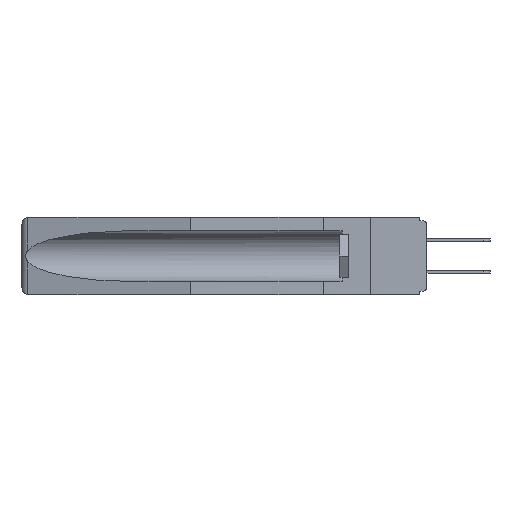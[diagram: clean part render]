
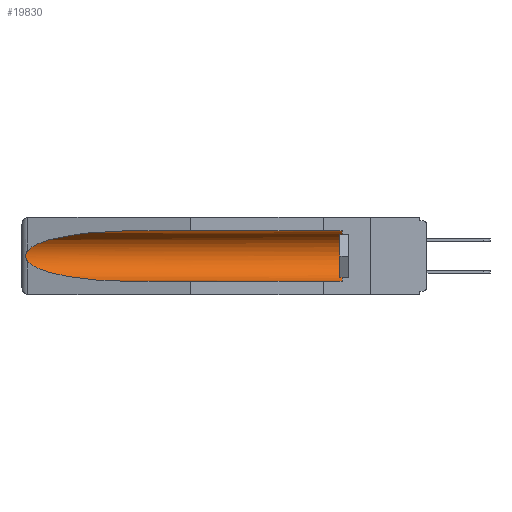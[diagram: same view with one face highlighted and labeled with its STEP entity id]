
A CAD part, left-side view. The second image highlights one B-rep face of the part: STEP entity #19830.
In plain terms, the highlighted cylindrical face has radius 2.857 mm (diameter 5.715 mm), a partial arc.
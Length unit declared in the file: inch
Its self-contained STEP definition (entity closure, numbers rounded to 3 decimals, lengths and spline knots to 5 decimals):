
#35 = CARTESIAN_POINT ( 'NONE',  ( 0.26655, 1.53094, -0.18657 ) ) ;
#414 = CYLINDRICAL_SURFACE ( 'NONE', #18750, 0.1125 ) ;
#430 = B_SPLINE_CURVE_WITH_KNOTS ( 'NONE', 3,
 ( #4669, #11144, #17852, #14540, #1374, #9643, #8009, #35, #12796, #11447 ),
 .UNSPECIFIED., .F., .F.,
 ( 4, 2, 2, 2, 4 ),
 ( 0., 0.00029, 0.00058, 0.00087, 0.00117 ),
 .UNSPECIFIED. ) ;
#1374 = CARTESIAN_POINT ( 'NONE',  ( 0.2675, 1.53308, -0.16763 ) ) ;
#1509 =( BOUNDED_CURVE ( )  B_SPLINE_CURVE ( 3, ( #13506, #6968, #18160, #20005 ),
 .UNSPECIFIED., .F., .F. ) 
 B_SPLINE_CURVE_WITH_KNOTS ( ( 4, 4 ),
 ( 4.71239, 6.08839 ),
 .UNSPECIFIED. ) 
 CURVE ( )  GEOMETRIC_REPRESENTATION_ITEM ( )  RATIONAL_B_SPLINE_CURVE ( ( 1., 0.848, 0.848, 1. ) ) 
 REPRESENTATION_ITEM ( '' )  );
#1814 = DIRECTION ( 'NONE',  ( 0., 1., 0. ) ) ;
#2579 = VERTEX_POINT ( 'NONE', #17797 ) ;
#2738 = ORIENTED_EDGE ( 'NONE', *, *, #10121, .T. ) ;
#2760 = EDGE_CURVE ( 'NONE', #20388, #2579, #17540, .T. ) ;
#4669 = CARTESIAN_POINT ( 'NONE',  ( 0.26537, 1.52718, -0.14972 ) ) ;
#5273 = ORIENTED_EDGE ( 'NONE', *, *, #15916, .F. ) ;
#5324 = DIRECTION ( 'NONE',  ( 0., 1., 0. ) ) ;
#5641 = CARTESIAN_POINT ( 'NONE',  ( 0.21114, 1.30732, -0.284 ) ) ;
#6081 = EDGE_CURVE ( 'NONE', #13293, #14736, #18174, .T. ) ;
#6417 = CARTESIAN_POINT ( 'NONE',  ( 0.26537, 1.52718, -0.14972 ) ) ;
#6472 = DIRECTION ( 'NONE',  ( 0., 0., 1. ) ) ;
#6864 = EDGE_CURVE ( 'NONE', #2579, #7585, #1509, .T. ) ;
#6968 = CARTESIAN_POINT ( 'NONE',  ( 0.21114, 1.30732, -0.059 ) ) ;
#7219 = CARTESIAN_POINT ( 'NONE',  ( 0.26537, 1.52718, -0.19328 ) ) ;
#7238 = LINE ( 'NONE', #16755, #11346 ) ;
#7585 = VERTEX_POINT ( 'NONE', #6417 ) ;
#7949 = DIRECTION ( 'NONE',  ( 0., 1., 0. ) ) ;
#8009 = CARTESIAN_POINT ( 'NONE',  ( 0.2673, 1.53269, -0.17917 ) ) ;
#8137 = ORIENTED_EDGE ( 'NONE', *, *, #6081, .T. ) ;
#8291 = CARTESIAN_POINT ( 'NONE',  ( 0.155, 0.126, -0.059 ) ) ;
#8417 = VECTOR ( 'NONE', #1814, 39.37008 ) ;
#8985 = ORIENTED_EDGE ( 'NONE', *, *, #6864, .T. ) ;
#9299 = CARTESIAN_POINT ( 'NONE',  ( 0.155, -0.30754, -0.1715 ) ) ;
#9643 = CARTESIAN_POINT ( 'NONE',  ( 0.2675, 1.53308, -0.17534 ) ) ;
#10121 = EDGE_CURVE ( 'NONE', #7585, #13293, #430, .T. ) ;
#10129 = CARTESIAN_POINT ( 'NONE',  ( 0.155, 0.126, -0.1715 ) ) ;
#10698 = CARTESIAN_POINT ( 'NONE',  ( 0.155, 0.126, -0.284 ) ) ;
#11144 = CARTESIAN_POINT ( 'NONE',  ( 0.26597, 1.52961, -0.15275 ) ) ;
#11211 = EDGE_LOOP ( 'NONE', ( #8985, #2738, #8137, #5273, #18683, #17648 ) ) ;
#11346 = VECTOR ( 'NONE', #5324, 39.37008 ) ;
#11447 = CARTESIAN_POINT ( 'NONE',  ( 0.26537, 1.52718, -0.19328 ) ) ;
#12330 = CARTESIAN_POINT ( 'NONE',  ( 0.26537, 1.52718, -0.19328 ) ) ;
#12765 = EDGE_CURVE ( 'NONE', #13415, #20388, #16172, .T. ) ;
#12796 = CARTESIAN_POINT ( 'NONE',  ( 0.26597, 1.5296, -0.19026 ) ) ;
#13148 = AXIS2_PLACEMENT_3D ( 'NONE', #10129, #20111, #15157 ) ;
#13293 = VERTEX_POINT ( 'NONE', #7219 ) ;
#13415 = VERTEX_POINT ( 'NONE', #10698 ) ;
#13506 = CARTESIAN_POINT ( 'NONE',  ( 0.155, 1.07973, -0.059 ) ) ;
#13812 = CARTESIAN_POINT ( 'NONE',  ( 0.155, 1.07973, -0.284 ) ) ;
#14540 = CARTESIAN_POINT ( 'NONE',  ( 0.2673, 1.5327, -0.16383 ) ) ;
#14656 = CARTESIAN_POINT ( 'NONE',  ( 0.155, 1.07973, -0.284 ) ) ;
#14736 = VERTEX_POINT ( 'NONE', #14656 ) ;
#15157 = DIRECTION ( 'NONE',  ( 0., 0., 1. ) ) ;
#15381 = CARTESIAN_POINT ( 'NONE',  ( 0.25451, 1.48313, -0.24835 ) ) ;
#15916 = EDGE_CURVE ( 'NONE', #13415, #14736, #7238, .T. ) ;
#16172 = CIRCLE ( 'NONE', #13148, 0.1125 ) ;
#16755 = CARTESIAN_POINT ( 'NONE',  ( 0.155, -0.30754, -0.284 ) ) ;
#17540 = LINE ( 'NONE', #19860, #8417 ) ;
#17648 = ORIENTED_EDGE ( 'NONE', *, *, #2760, .T. ) ;
#17797 = CARTESIAN_POINT ( 'NONE',  ( 0.155, 1.07973, -0.059 ) ) ;
#17852 = CARTESIAN_POINT ( 'NONE',  ( 0.26654, 1.53092, -0.15636 ) ) ;
#18160 = CARTESIAN_POINT ( 'NONE',  ( 0.25451, 1.48313, -0.09465 ) ) ;
#18174 =( BOUNDED_CURVE ( )  B_SPLINE_CURVE ( 3, ( #12330, #15381, #5641, #13812 ),
 .UNSPECIFIED., .F., .F. ) 
 B_SPLINE_CURVE_WITH_KNOTS ( ( 4, 4 ),
 ( 0.1948, 1.5708 ),
 .UNSPECIFIED. ) 
 CURVE ( )  GEOMETRIC_REPRESENTATION_ITEM ( )  RATIONAL_B_SPLINE_CURVE ( ( 1., 0.848, 0.848, 1. ) ) 
 REPRESENTATION_ITEM ( '' )  );
#18683 = ORIENTED_EDGE ( 'NONE', *, *, #12765, .T. ) ;
#18750 = AXIS2_PLACEMENT_3D ( 'NONE', #9299, #7949, #6472 ) ;
#19830 = ADVANCED_FACE ( 'NONE', ( #21028 ), #414, .F. ) ;
#19860 = CARTESIAN_POINT ( 'NONE',  ( 0.155, -0.30754, -0.059 ) ) ;
#20005 = CARTESIAN_POINT ( 'NONE',  ( 0.26537, 1.52718, -0.14972 ) ) ;
#20111 = DIRECTION ( 'NONE',  ( 0., -1., 0. ) ) ;
#20388 = VERTEX_POINT ( 'NONE', #8291 ) ;
#21028 = FACE_OUTER_BOUND ( 'NONE', #11211, .T. ) ;
